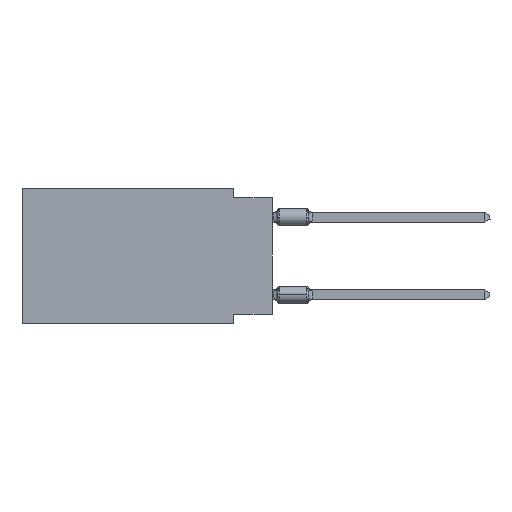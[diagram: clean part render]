
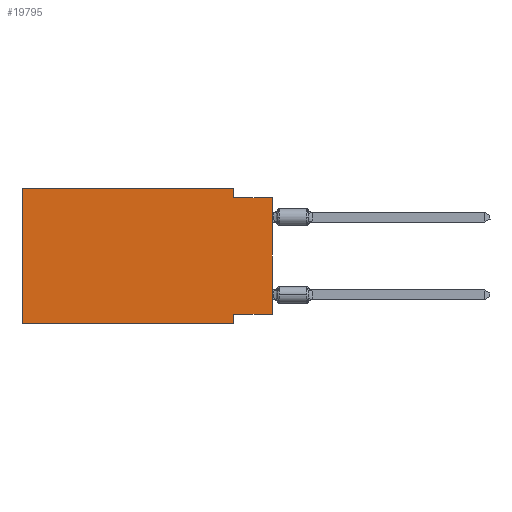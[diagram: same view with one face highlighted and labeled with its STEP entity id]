
A CAD part, left-side view. The second image highlights one B-rep face of the part: STEP entity #19795.
In plain terms, the highlighted planar face has unit normal (-1, 0, 0).
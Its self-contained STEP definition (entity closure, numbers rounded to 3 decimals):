
#503 = VECTOR ( 'NONE', #34916, 1000. ) ;
#654 = PLANE ( 'NONE',  #23923 ) ;
#706 = CARTESIAN_POINT ( 'NONE',  ( 0., 2.54, -8.255 ) ) ;
#3831 = VERTEX_POINT ( 'NONE', #6478 ) ;
#3926 = LINE ( 'NONE', #18427, #17164 ) ;
#3971 = EDGE_CURVE ( 'NONE', #31002, #32973, #19931, .T. ) ;
#4640 = CARTESIAN_POINT ( 'NONE',  ( 0., 2.54, -8.89 ) ) ;
#5490 = VECTOR ( 'NONE', #24919, 1000. ) ;
#5999 = EDGE_CURVE ( 'NONE', #9086, #3831, #31918, .T. ) ;
#6202 = VECTOR ( 'NONE', #37743, 1000. ) ;
#6478 = CARTESIAN_POINT ( 'NONE',  ( 0., 2.54, 0. ) ) ;
#6795 = CARTESIAN_POINT ( 'NONE',  ( 0., 16.383, 0. ) ) ;
#8479 = EDGE_CURVE ( 'NONE', #8788, #31002, #23319, .T. ) ;
#8701 = LINE ( 'NONE', #36469, #37719 ) ;
#8788 = VERTEX_POINT ( 'NONE', #22096 ) ;
#9086 = VERTEX_POINT ( 'NONE', #11598 ) ;
#9583 = LINE ( 'NONE', #19238, #6202 ) ;
#10476 = EDGE_CURVE ( 'NONE', #25814, #9086, #9583, .T. ) ;
#10809 = CARTESIAN_POINT ( 'NONE',  ( 0., 2.54, 0. ) ) ;
#11098 = ORIENTED_EDGE ( 'NONE', *, *, #24145, .F. ) ;
#11598 = CARTESIAN_POINT ( 'NONE',  ( 0., 16.383, 0. ) ) ;
#12296 = VERTEX_POINT ( 'NONE', #29210 ) ;
#12910 = DIRECTION ( 'NONE',  ( 1., 0., 0. ) ) ;
#13207 = ORIENTED_EDGE ( 'NONE', *, *, #31238, .T. ) ;
#15472 = CARTESIAN_POINT ( 'NONE',  ( 0., 2.54, -0.635 ) ) ;
#17164 = VECTOR ( 'NONE', #30890, 1000. ) ;
#17255 = DIRECTION ( 'NONE',  ( 0., 0., -1. ) ) ;
#17959 = DIRECTION ( 'NONE',  ( 0., 0., 1. ) ) ;
#18042 = ORIENTED_EDGE ( 'NONE', *, *, #8479, .F. ) ;
#18427 = CARTESIAN_POINT ( 'NONE',  ( 0., 0., -0.635 ) ) ;
#18478 = CARTESIAN_POINT ( 'NONE',  ( 0., 16.383, -8.89 ) ) ;
#19238 = CARTESIAN_POINT ( 'NONE',  ( 0., 16.383, 0. ) ) ;
#19305 = ORIENTED_EDGE ( 'NONE', *, *, #3971, .F. ) ;
#19309 = ORIENTED_EDGE ( 'NONE', *, *, #37911, .F. ) ;
#19795 = ADVANCED_FACE ( 'NONE', ( #31219 ), #654, .F. ) ;
#19931 = LINE ( 'NONE', #4640, #37162 ) ;
#22096 = CARTESIAN_POINT ( 'NONE',  ( 0., 0., -8.255 ) ) ;
#23319 = LINE ( 'NONE', #38426, #30460 ) ;
#23715 = ORIENTED_EDGE ( 'NONE', *, *, #10476, .F. ) ;
#23923 = AXIS2_PLACEMENT_3D ( 'NONE', #24578, #12910, #34029 ) ;
#24145 = EDGE_CURVE ( 'NONE', #27255, #12296, #3926, .T. ) ;
#24578 = CARTESIAN_POINT ( 'NONE',  ( 0., 16.383, 0. ) ) ;
#24919 = DIRECTION ( 'NONE',  ( 0., -1., 0. ) ) ;
#25756 = DIRECTION ( 'NONE',  ( 0., 1., 0. ) ) ;
#25814 = VERTEX_POINT ( 'NONE', #33871 ) ;
#26878 = EDGE_LOOP ( 'NONE', ( #13207, #11098, #19309, #31160, #23715, #34996, #19305, #18042 ) ) ;
#27255 = VERTEX_POINT ( 'NONE', #15472 ) ;
#29210 = CARTESIAN_POINT ( 'NONE',  ( 0., 0., -0.635 ) ) ;
#30460 = VECTOR ( 'NONE', #25756, 1000. ) ;
#30890 = DIRECTION ( 'NONE',  ( 0., -1., 0. ) ) ;
#31002 = VERTEX_POINT ( 'NONE', #706 ) ;
#31160 = ORIENTED_EDGE ( 'NONE', *, *, #5999, .F. ) ;
#31219 = FACE_OUTER_BOUND ( 'NONE', #26878, .T. ) ;
#31238 = EDGE_CURVE ( 'NONE', #8788, #12296, #8701, .T. ) ;
#31841 = VECTOR ( 'NONE', #17255, 1000. ) ;
#31918 = LINE ( 'NONE', #6795, #503 ) ;
#32973 = VERTEX_POINT ( 'NONE', #38008 ) ;
#33740 = LINE ( 'NONE', #18478, #5490 ) ;
#33871 = CARTESIAN_POINT ( 'NONE',  ( 0., 16.383, -8.89 ) ) ;
#34029 = DIRECTION ( 'NONE',  ( 0., 0., -1. ) ) ;
#34916 = DIRECTION ( 'NONE',  ( 0., -1., 0. ) ) ;
#34996 = ORIENTED_EDGE ( 'NONE', *, *, #39121, .T. ) ;
#35940 = LINE ( 'NONE', #10809, #31841 ) ;
#36469 = CARTESIAN_POINT ( 'NONE',  ( 0., 0., 0. ) ) ;
#37162 = VECTOR ( 'NONE', #37849, 1000. ) ;
#37719 = VECTOR ( 'NONE', #17959, 1000. ) ;
#37743 = DIRECTION ( 'NONE',  ( 0., 0., 1. ) ) ;
#37849 = DIRECTION ( 'NONE',  ( 0., 0., -1. ) ) ;
#37911 = EDGE_CURVE ( 'NONE', #3831, #27255, #35940, .T. ) ;
#38008 = CARTESIAN_POINT ( 'NONE',  ( 0., 2.54, -8.89 ) ) ;
#38426 = CARTESIAN_POINT ( 'NONE',  ( 0., 0., -8.255 ) ) ;
#39121 = EDGE_CURVE ( 'NONE', #25814, #32973, #33740, .T. ) ;
